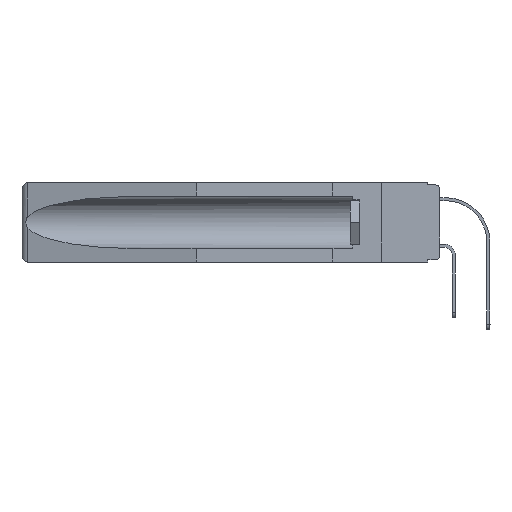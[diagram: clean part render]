
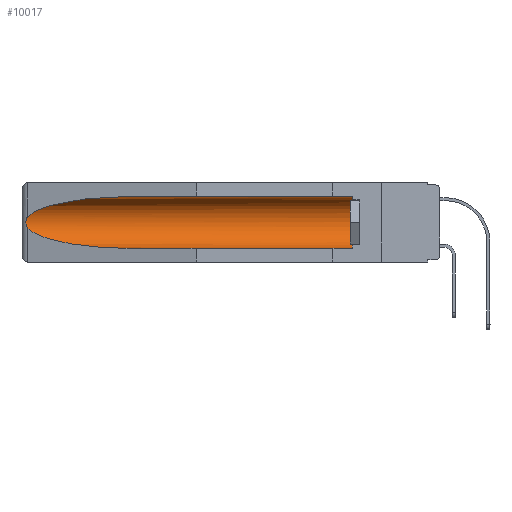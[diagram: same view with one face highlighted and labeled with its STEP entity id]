
A CAD part, left-side view. The second image highlights one B-rep face of the part: STEP entity #10017.
In plain terms, the highlighted cylindrical face has radius 2.857 mm (diameter 5.715 mm), a partial arc.
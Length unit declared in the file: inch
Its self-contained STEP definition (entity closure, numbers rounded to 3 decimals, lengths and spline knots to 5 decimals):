
#172 = EDGE_CURVE ( 'NONE', #2176, #12816, #10537, .T. ) ;
#447 = VECTOR ( 'NONE', #9949, 39.37008 ) ;
#555 = CARTESIAN_POINT ( 'NONE',  ( 0.26537, 1.52718, -0.19328 ) ) ;
#687 = ORIENTED_EDGE ( 'NONE', *, *, #3489, .T. ) ;
#1624 = CARTESIAN_POINT ( 'NONE',  ( 0.25451, 1.48313, -0.24835 ) ) ;
#1660 = ORIENTED_EDGE ( 'NONE', *, *, #15441, .T. ) ;
#1744 = CARTESIAN_POINT ( 'NONE',  ( 0.21114, 1.30732, -0.059 ) ) ;
#2176 = VERTEX_POINT ( 'NONE', #3956 ) ;
#3489 = EDGE_CURVE ( 'NONE', #5442, #2176, #15612, .T. ) ;
#3626 = FACE_OUTER_BOUND ( 'NONE', #5093, .T. ) ;
#3793 = DIRECTION ( 'NONE',  ( 0., 1., 0. ) ) ;
#3956 = CARTESIAN_POINT ( 'NONE',  ( 0.155, 0.126, -0.059 ) ) ;
#5016 = EDGE_CURVE ( 'NONE', #12816, #5548, #15656, .T. ) ;
#5051 = VERTEX_POINT ( 'NONE', #15304 ) ;
#5093 = EDGE_LOOP ( 'NONE', ( #7255, #1660, #11755, #16231, #687, #12502 ) ) ;
#5273 = CARTESIAN_POINT ( 'NONE',  ( 0.26537, 1.52718, -0.19328 ) ) ;
#5366 = CARTESIAN_POINT ( 'NONE',  ( 0.2675, 1.53308, -0.17534 ) ) ;
#5415 = VECTOR ( 'NONE', #3793, 39.37008 ) ;
#5442 = VERTEX_POINT ( 'NONE', #5799 ) ;
#5548 = VERTEX_POINT ( 'NONE', #7297 ) ;
#5584 = B_SPLINE_CURVE_WITH_KNOTS ( 'NONE', 3,
 ( #8097, #11990, #6774, #13412, #10671, #5366, #6856, #13594, #12252, #5273 ),
 .UNSPECIFIED., .F., .F.,
 ( 4, 2, 2, 2, 4 ),
 ( 0., 0.00029, 0.00058, 0.00087, 0.00117 ),
 .UNSPECIFIED. ) ;
#5646 = DIRECTION ( 'NONE',  ( 0., -1., 0. ) ) ;
#5717 = CARTESIAN_POINT ( 'NONE',  ( 0.155, -0.30754, -0.284 ) ) ;
#5799 = CARTESIAN_POINT ( 'NONE',  ( 0.155, 0.126, -0.284 ) ) ;
#5966 = CARTESIAN_POINT ( 'NONE',  ( 0.21114, 1.30732, -0.284 ) ) ;
#6774 = CARTESIAN_POINT ( 'NONE',  ( 0.26654, 1.53092, -0.15636 ) ) ;
#6856 = CARTESIAN_POINT ( 'NONE',  ( 0.2673, 1.53269, -0.17917 ) ) ;
#7032 = CARTESIAN_POINT ( 'NONE',  ( 0.155, 1.07973, -0.284 ) ) ;
#7139 = CARTESIAN_POINT ( 'NONE',  ( 0.25451, 1.48313, -0.09465 ) ) ;
#7255 = ORIENTED_EDGE ( 'NONE', *, *, #5016, .T. ) ;
#7297 = CARTESIAN_POINT ( 'NONE',  ( 0.26537, 1.52718, -0.14972 ) ) ;
#8097 = CARTESIAN_POINT ( 'NONE',  ( 0.26537, 1.52718, -0.14972 ) ) ;
#8938 = CARTESIAN_POINT ( 'NONE',  ( 0.26537, 1.52718, -0.19328 ) ) ;
#9949 = DIRECTION ( 'NONE',  ( 0., 1., 0. ) ) ;
#10017 = ADVANCED_FACE ( 'NONE', ( #3626 ), #11511, .F. ) ;
#10503 = AXIS2_PLACEMENT_3D ( 'NONE', #13439, #5646, #13619 ) ;
#10537 = LINE ( 'NONE', #15954, #5415 ) ;
#10539 = EDGE_CURVE ( 'NONE', #11621, #5051, #11449, .T. ) ;
#10671 = CARTESIAN_POINT ( 'NONE',  ( 0.2675, 1.53308, -0.16763 ) ) ;
#11449 =( BOUNDED_CURVE ( )  B_SPLINE_CURVE ( 3, ( #555, #1624, #5966, #7032 ),
 .UNSPECIFIED., .F., .F. ) 
 B_SPLINE_CURVE_WITH_KNOTS ( ( 4, 4 ),
 ( 0.1948, 1.5708 ),
 .UNSPECIFIED. ) 
 CURVE ( )  GEOMETRIC_REPRESENTATION_ITEM ( )  RATIONAL_B_SPLINE_CURVE ( ( 1., 0.848, 0.848, 1. ) ) 
 REPRESENTATION_ITEM ( '' )  );
#11511 = CYLINDRICAL_SURFACE ( 'NONE', #16332, 0.1125 ) ;
#11621 = VERTEX_POINT ( 'NONE', #8938 ) ;
#11755 = ORIENTED_EDGE ( 'NONE', *, *, #10539, .T. ) ;
#11857 = DIRECTION ( 'NONE',  ( 0., 1., 0. ) ) ;
#11990 = CARTESIAN_POINT ( 'NONE',  ( 0.26597, 1.52961, -0.15275 ) ) ;
#12252 = CARTESIAN_POINT ( 'NONE',  ( 0.26597, 1.5296, -0.19026 ) ) ;
#12434 = CARTESIAN_POINT ( 'NONE',  ( 0.155, 1.07973, -0.059 ) ) ;
#12502 = ORIENTED_EDGE ( 'NONE', *, *, #172, .T. ) ;
#12640 = CARTESIAN_POINT ( 'NONE',  ( 0.26537, 1.52718, -0.14972 ) ) ;
#12805 = CARTESIAN_POINT ( 'NONE',  ( 0.155, 1.07973, -0.059 ) ) ;
#12816 = VERTEX_POINT ( 'NONE', #12434 ) ;
#13101 = DIRECTION ( 'NONE',  ( 0., 0., 1. ) ) ;
#13412 = CARTESIAN_POINT ( 'NONE',  ( 0.2673, 1.5327, -0.16383 ) ) ;
#13439 = CARTESIAN_POINT ( 'NONE',  ( 0.155, 0.126, -0.1715 ) ) ;
#13594 = CARTESIAN_POINT ( 'NONE',  ( 0.26655, 1.53094, -0.18657 ) ) ;
#13619 = DIRECTION ( 'NONE',  ( 0., 0., 1. ) ) ;
#15304 = CARTESIAN_POINT ( 'NONE',  ( 0.155, 1.07973, -0.284 ) ) ;
#15441 = EDGE_CURVE ( 'NONE', #5548, #11621, #5584, .T. ) ;
#15612 = CIRCLE ( 'NONE', #10503, 0.1125 ) ;
#15656 =( BOUNDED_CURVE ( )  B_SPLINE_CURVE ( 3, ( #12805, #1744, #7139, #12640 ),
 .UNSPECIFIED., .F., .F. ) 
 B_SPLINE_CURVE_WITH_KNOTS ( ( 4, 4 ),
 ( 4.71239, 6.08839 ),
 .UNSPECIFIED. ) 
 CURVE ( )  GEOMETRIC_REPRESENTATION_ITEM ( )  RATIONAL_B_SPLINE_CURVE ( ( 1., 0.848, 0.848, 1. ) ) 
 REPRESENTATION_ITEM ( '' )  );
#15954 = CARTESIAN_POINT ( 'NONE',  ( 0.155, -0.30754, -0.059 ) ) ;
#16231 = ORIENTED_EDGE ( 'NONE', *, *, #16918, .F. ) ;
#16332 = AXIS2_PLACEMENT_3D ( 'NONE', #17011, #11857, #13101 ) ;
#16445 = LINE ( 'NONE', #5717, #447 ) ;
#16918 = EDGE_CURVE ( 'NONE', #5442, #5051, #16445, .T. ) ;
#17011 = CARTESIAN_POINT ( 'NONE',  ( 0.155, -0.30754, -0.1715 ) ) ;
